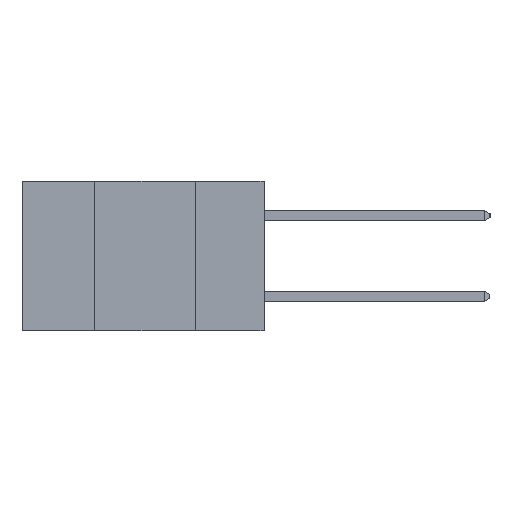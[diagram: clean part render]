
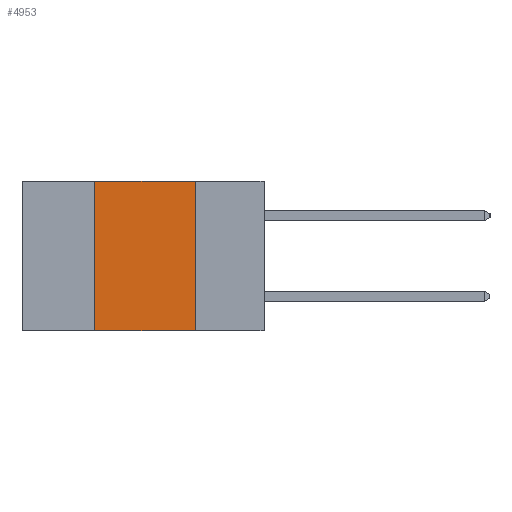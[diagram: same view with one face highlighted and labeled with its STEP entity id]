
A CAD part, left-side view. The second image highlights one B-rep face of the part: STEP entity #4953.
In plain terms, the highlighted planar face has unit normal (-1, 0, 0).
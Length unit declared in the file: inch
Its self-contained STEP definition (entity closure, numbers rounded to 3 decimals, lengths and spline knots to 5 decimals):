
#596 = CARTESIAN_POINT ( 'NONE',  ( 0., 0.6, -0.37 ) ) ;
#740 = CARTESIAN_POINT ( 'NONE',  ( 0., 0.17, 0. ) ) ;
#1083 = ORIENTED_EDGE ( 'NONE', *, *, #10414, .F. ) ;
#1877 = VECTOR ( 'NONE', #10999, 39.37008 ) ;
#2854 = LINE ( 'NONE', #2924, #3519 ) ;
#2856 = ORIENTED_EDGE ( 'NONE', *, *, #14269, .T. ) ;
#2924 = CARTESIAN_POINT ( 'NONE',  ( 0., 0.17, -0.37 ) ) ;
#2977 = CARTESIAN_POINT ( 'NONE',  ( 0., 0.42, 0. ) ) ;
#3262 = CARTESIAN_POINT ( 'NONE',  ( 0., 0.42, -0.37 ) ) ;
#3323 = AXIS2_PLACEMENT_3D ( 'NONE', #12736, #11820, #11744 ) ;
#3466 = FACE_OUTER_BOUND ( 'NONE', #4828, .T. ) ;
#3519 = VECTOR ( 'NONE', #7483, 39.37008 ) ;
#4717 = EDGE_CURVE ( 'NONE', #8148, #7869, #2854, .T. ) ;
#4828 = EDGE_LOOP ( 'NONE', ( #9703, #14000, #1083, #2856 ) ) ;
#4953 = ADVANCED_FACE ( 'NONE', ( #3466 ), #8028, .F. ) ;
#5546 = LINE ( 'NONE', #13576, #9017 ) ;
#5702 = VERTEX_POINT ( 'NONE', #2977 ) ;
#6345 = VERTEX_POINT ( 'NONE', #3262 ) ;
#7483 = DIRECTION ( 'NONE',  ( 0., 0., -1. ) ) ;
#7869 = VERTEX_POINT ( 'NONE', #14498 ) ;
#8028 = PLANE ( 'NONE',  #3323 ) ;
#8148 = VERTEX_POINT ( 'NONE', #740 ) ;
#8986 = DIRECTION ( 'NONE',  ( 0., -1., 0. ) ) ;
#9017 = VECTOR ( 'NONE', #8986, 39.37008 ) ;
#9703 = ORIENTED_EDGE ( 'NONE', *, *, #4717, .F. ) ;
#10414 = EDGE_CURVE ( 'NONE', #6345, #5702, #11575, .T. ) ;
#10428 = CARTESIAN_POINT ( 'NONE',  ( 0., 0.42, -0.37 ) ) ;
#10921 = LINE ( 'NONE', #596, #1877 ) ;
#10999 = DIRECTION ( 'NONE',  ( 0., -1., 0. ) ) ;
#11575 = LINE ( 'NONE', #10428, #14625 ) ;
#11744 = DIRECTION ( 'NONE',  ( 0., 0., -1. ) ) ;
#11820 = DIRECTION ( 'NONE',  ( 1., 0., 0. ) ) ;
#12736 = CARTESIAN_POINT ( 'NONE',  ( 0., 0.6, 0. ) ) ;
#13576 = CARTESIAN_POINT ( 'NONE',  ( 0., 0.6, 0. ) ) ;
#13905 = DIRECTION ( 'NONE',  ( 0., 0., 1. ) ) ;
#14000 = ORIENTED_EDGE ( 'NONE', *, *, #14717, .F. ) ;
#14269 = EDGE_CURVE ( 'NONE', #6345, #7869, #10921, .T. ) ;
#14498 = CARTESIAN_POINT ( 'NONE',  ( 0., 0.17, -0.37 ) ) ;
#14625 = VECTOR ( 'NONE', #13905, 39.37008 ) ;
#14717 = EDGE_CURVE ( 'NONE', #5702, #8148, #5546, .T. ) ;
